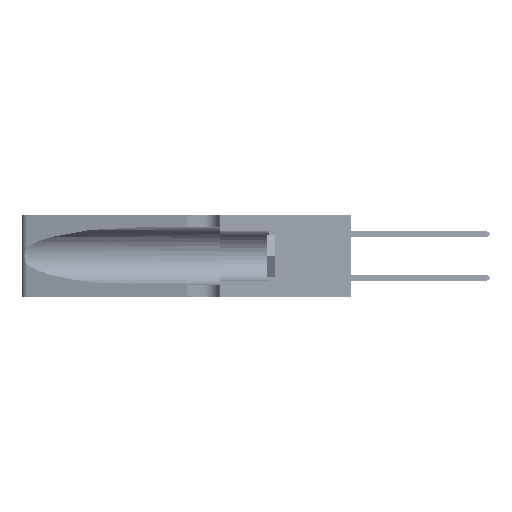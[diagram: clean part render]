
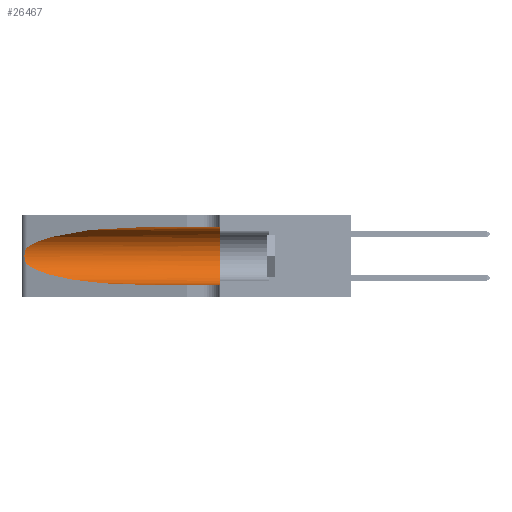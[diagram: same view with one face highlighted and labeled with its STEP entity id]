
A CAD part, left-side view. The second image highlights one B-rep face of the part: STEP entity #26467.
In plain terms, the highlighted cylindrical face has radius 3.308 mm (diameter 6.617 mm), a partial arc.
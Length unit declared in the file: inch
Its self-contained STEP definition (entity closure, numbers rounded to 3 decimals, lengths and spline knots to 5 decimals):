
#1462 = EDGE_CURVE ( 'NONE', #24086, #8345, #38622, .T. ) ;
#1644 = CARTESIAN_POINT ( 'NONE',  ( 0.1305, 0.72297, 0.05475 ) ) ;
#2520 = CARTESIAN_POINT ( 'NONE',  ( 0.1305, 0.35, 0.185 ) ) ;
#2564 = CARTESIAN_POINT ( 'NONE',  ( 0.25639, 1.23184, 0.21858 ) ) ;
#2731 = CARTESIAN_POINT ( 'NONE',  ( 0.25787, 1.23484, 0.2124 ) ) ;
#3135 = ORIENTED_EDGE ( 'NONE', *, *, #50610, .T. ) ;
#7029 = CARTESIAN_POINT ( 'NONE',  ( 0.1305, 0.35, 0.31525 ) ) ;
#7728 = AXIS2_PLACEMENT_3D ( 'NONE', #32255, #28615, #40319 ) ;
#8345 = VERTEX_POINT ( 'NONE', #11374 ) ;
#8949 = AXIS2_PLACEMENT_3D ( 'NONE', #2520, #50205, #15625 ) ;
#9466 = CARTESIAN_POINT ( 'NONE',  ( 0.2373, 1.15595, 0.08982 ) ) ;
#10288 = CYLINDRICAL_SURFACE ( 'NONE', #7728, 0.13025 ) ;
#10583 = DIRECTION ( 'NONE',  ( 0., -1., 0. ) ) ;
#10694 = CARTESIAN_POINT ( 'NONE',  ( 0.25487, 1.22718, 0.22369 ) ) ;
#11214 = ORIENTED_EDGE ( 'NONE', *, *, #35934, .T. ) ;
#11374 = CARTESIAN_POINT ( 'NONE',  ( 0.25487, 1.22718, 0.14631 ) ) ;
#11724 = VERTEX_POINT ( 'NONE', #37667 ) ;
#11822 = LINE ( 'NONE', #50313, #20435 ) ;
#13419 = LINE ( 'NONE', #42218, #42589 ) ;
#14336 = CARTESIAN_POINT ( 'NONE',  ( 0.25555, 1.22993, 0.14849 ) ) ;
#14786 = ORIENTED_EDGE ( 'NONE', *, *, #35852, .T. ) ;
#14886 = ORIENTED_EDGE ( 'NONE', *, *, #47191, .F. ) ;
#15625 = DIRECTION ( 'NONE',  ( 0., 0., 1. ) ) ;
#20435 = VECTOR ( 'NONE', #10583, 39.37008 ) ;
#22100 = CARTESIAN_POINT ( 'NONE',  ( 0.26018, 1.23835, 0.19895 ) ) ;
#22605 = CARTESIAN_POINT ( 'NONE',  ( 0.26075, 1.23896, 0.178 ) ) ;
#24086 = VERTEX_POINT ( 'NONE', #26720 ) ;
#24551 = ORIENTED_EDGE ( 'NONE', *, *, #29853, .F. ) ;
#26076 = CARTESIAN_POINT ( 'NONE',  ( 0.25555, 1.22994, 0.2215 ) ) ;
#26390 = CARTESIAN_POINT ( 'NONE',  ( 0.2373, 1.15595, 0.28018 ) ) ;
#26467 = ADVANCED_FACE ( 'NONE', ( #47520 ), #10288, .F. ) ;
#26557 = CARTESIAN_POINT ( 'NONE',  ( 0.25487, 1.22718, 0.22369 ) ) ;
#26720 = CARTESIAN_POINT ( 'NONE',  ( 0.25487, 1.22718, 0.22369 ) ) ;
#28163 = VERTEX_POINT ( 'NONE', #7029 ) ;
#28447 = CIRCLE ( 'NONE', #8949, 0.13025 ) ;
#28615 = DIRECTION ( 'NONE',  ( 0., -1., 0. ) ) ;
#28869 = CARTESIAN_POINT ( 'NONE',  ( 0.1305, 0.35, 0.05475 ) ) ;
#28958 =( BOUNDED_CURVE ( )  B_SPLINE_CURVE ( 3, ( #46242, #41737, #26390, #26557 ),
 .UNSPECIFIED., .F., .F. ) 
 B_SPLINE_CURVE_WITH_KNOTS ( ( 4, 4 ),
 ( 1.5708, 2.84003 ),
 .UNSPECIFIED. ) 
 CURVE ( )  GEOMETRIC_REPRESENTATION_ITEM ( )  RATIONAL_B_SPLINE_CURVE ( ( 1., 0.87, 0.87, 1. ) ) 
 REPRESENTATION_ITEM ( '' )  );
#29853 = EDGE_CURVE ( 'NONE', #28163, #30813, #28447, .T. ) ;
#30385 = CARTESIAN_POINT ( 'NONE',  ( 0.26017, 1.23833, 0.17102 ) ) ;
#30813 = VERTEX_POINT ( 'NONE', #28869 ) ;
#32255 = CARTESIAN_POINT ( 'NONE',  ( 0.1305, 1.61858, 0.185 ) ) ;
#33894 = CARTESIAN_POINT ( 'NONE',  ( 0.25854, 1.2359, 0.20912 ) ) ;
#34063 = CARTESIAN_POINT ( 'NONE',  ( 0.25487, 1.22718, 0.14631 ) ) ;
#34238 = CARTESIAN_POINT ( 'NONE',  ( 0.25639, 1.23186, 0.15144 ) ) ;
#35283 = VERTEX_POINT ( 'NONE', #48973 ) ;
#35852 = EDGE_CURVE ( 'NONE', #8345, #35283, #37289, .T. ) ;
#35934 = EDGE_CURVE ( 'NONE', #35283, #30813, #13419, .T. ) ;
#37006 = ORIENTED_EDGE ( 'NONE', *, *, #1462, .T. ) ;
#37150 = CARTESIAN_POINT ( 'NONE',  ( 0.18966, 0.96281, 0.05475 ) ) ;
#37289 =( BOUNDED_CURVE ( )  B_SPLINE_CURVE ( 3, ( #49007, #9466, #37150, #1644 ),
 .UNSPECIFIED., .F., .F. ) 
 B_SPLINE_CURVE_WITH_KNOTS ( ( 4, 4 ),
 ( 3.44316, 4.71239 ),
 .UNSPECIFIED. ) 
 CURVE ( )  GEOMETRIC_REPRESENTATION_ITEM ( )  RATIONAL_B_SPLINE_CURVE ( ( 1., 0.87, 0.87, 1. ) ) 
 REPRESENTATION_ITEM ( '' )  );
#37667 = CARTESIAN_POINT ( 'NONE',  ( 0.1305, 0.72297, 0.31525 ) ) ;
#38432 = CARTESIAN_POINT ( 'NONE',  ( 0.25789, 1.23486, 0.15765 ) ) ;
#38622 = B_SPLINE_CURVE_WITH_KNOTS ( 'NONE', 3,
 ( #10694, #26076, #2564, #2731, #33894, #22100, #42276, #22605, #30385, #46096, #38432, #34238, #14336, #34063 ),
 .UNSPECIFIED., .F., .F.,
 ( 4, 2, 2, 2, 2, 2, 4 ),
 ( 0., 0.00027, 0.00053, 0.00107, 0.0016, 0.00187, 0.00214 ),
 .UNSPECIFIED. ) ;
#40319 = DIRECTION ( 'NONE',  ( 0., 0., -1. ) ) ;
#41737 = CARTESIAN_POINT ( 'NONE',  ( 0.18966, 0.96281, 0.31525 ) ) ;
#42218 = CARTESIAN_POINT ( 'NONE',  ( 0.1305, 1.61858, 0.05475 ) ) ;
#42276 = CARTESIAN_POINT ( 'NONE',  ( 0.26075, 1.23896, 0.19203 ) ) ;
#42589 = VECTOR ( 'NONE', #46041, 39.37008 ) ;
#45919 = EDGE_LOOP ( 'NONE', ( #3135, #37006, #14786, #11214, #24551, #14886 ) ) ;
#46041 = DIRECTION ( 'NONE',  ( 0., -1., 0. ) ) ;
#46096 = CARTESIAN_POINT ( 'NONE',  ( 0.25856, 1.23593, 0.16098 ) ) ;
#46242 = CARTESIAN_POINT ( 'NONE',  ( 0.1305, 0.72297, 0.31525 ) ) ;
#47191 = EDGE_CURVE ( 'NONE', #11724, #28163, #11822, .T. ) ;
#47520 = FACE_OUTER_BOUND ( 'NONE', #45919, .T. ) ;
#48973 = CARTESIAN_POINT ( 'NONE',  ( 0.1305, 0.72297, 0.05475 ) ) ;
#49007 = CARTESIAN_POINT ( 'NONE',  ( 0.25487, 1.22718, 0.14631 ) ) ;
#50205 = DIRECTION ( 'NONE',  ( 0., 1., 0. ) ) ;
#50313 = CARTESIAN_POINT ( 'NONE',  ( 0.1305, 1.61858, 0.31525 ) ) ;
#50610 = EDGE_CURVE ( 'NONE', #11724, #24086, #28958, .T. ) ;
